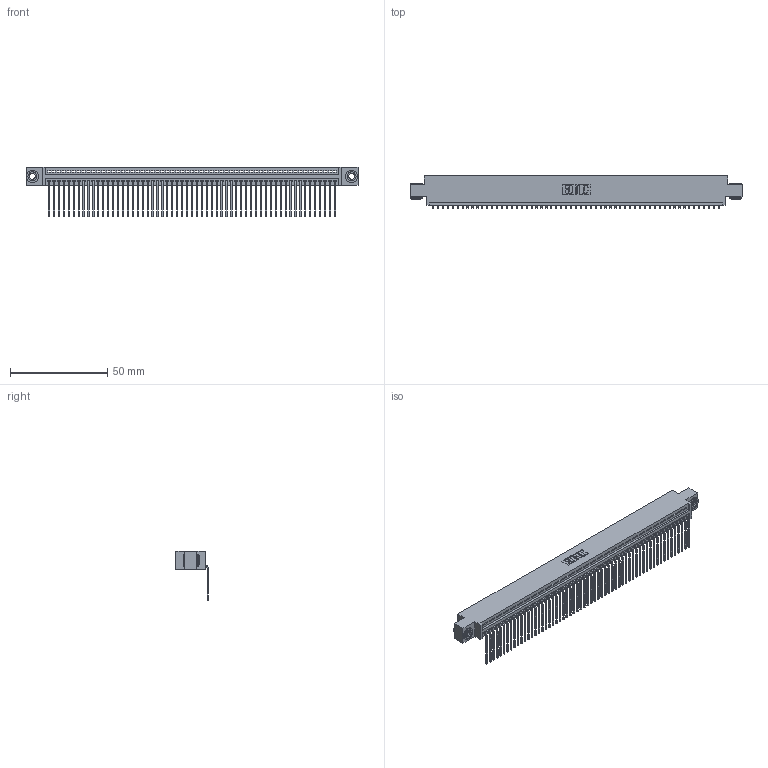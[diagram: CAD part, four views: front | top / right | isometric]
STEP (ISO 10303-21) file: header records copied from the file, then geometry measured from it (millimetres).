
FILE_DESCRIPTION (( 'STEP AP203' ), '1' );
FILE_NAME ('395-059-559-603.STEP', '2018-11-23T10:15:27', ( '' ), ( '' ), 'SwSTEP 2.0', 'SolidWorks 2016', '' );
FILE_SCHEMA (( 'CONFIG_CONTROL_DESIGN' ));
Length unit declared in the file: inch
Products named in the file (4): 345-250-002_345-250-002-102; 345 Part_0.170 Offset - 0.156 Dia-TH; 395-059-559-603; 345-292-001_558 559 Tail - 1
Assembly tree (62 placements, depth 2):
  395-059-559-603
    345 Part_0.170 Offset - 0.156 Dia-TH
    345-292-001_558 559 Tail - 1  x59
    345-250-002_345-250-002-102  x2
Bounding box: 171.07 x 16.75 x 25.53 mm (x, y, z)
Volume: 16490.2 mm3; surface area: 23641.1 mm2
Topology: 62 solids, 62 shells, 3708 faces, 11167 edges, 7362 vertices
Faces by surface type: plane 2572, cylinder 1128, cone 8
Entity records: 42982 total; most frequent: CARTESIAN_POINT 7424, ORIENTED_EDGE 7410, DIRECTION 6489, EDGE_CURVE 3705, VECTOR 3313, LINE 3313, VERTEX_POINT 2466, AXIS2_PLACEMENT_3D 1588
